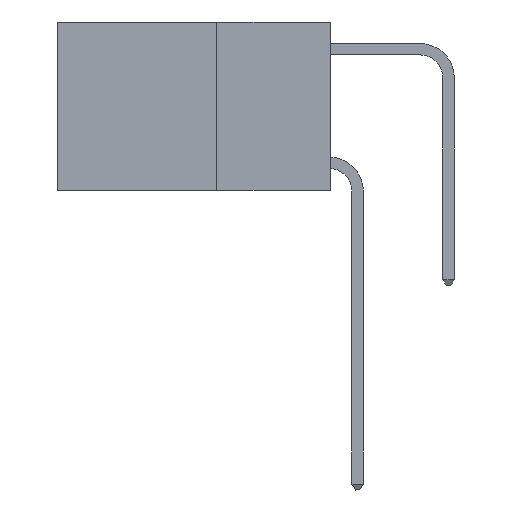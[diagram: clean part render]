
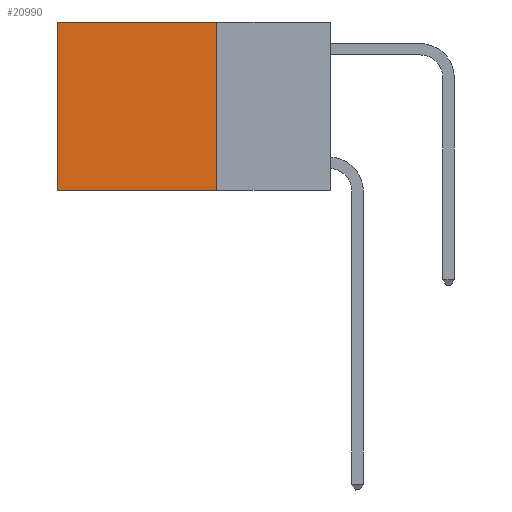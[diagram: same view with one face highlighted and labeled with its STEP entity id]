
A CAD part, left-side view. The second image highlights one B-rep face of the part: STEP entity #20990.
In plain terms, the highlighted planar face has unit normal (-1, 0, 0).
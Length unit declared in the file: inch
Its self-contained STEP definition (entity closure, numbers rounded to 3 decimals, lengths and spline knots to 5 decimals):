
#820 = CARTESIAN_POINT ( 'NONE',  ( 0.2625, 0.25, 0. ) ) ;
#863 = VECTOR ( 'NONE', #4095, 39.37008 ) ;
#1555 = PLANE ( 'NONE',  #19577 ) ;
#2429 = LINE ( 'NONE', #5740, #863 ) ;
#3528 = CARTESIAN_POINT ( 'NONE',  ( 0.2625, 0.6, 0. ) ) ;
#4095 = DIRECTION ( 'NONE',  ( 0., 0., -1. ) ) ;
#4632 = CARTESIAN_POINT ( 'NONE',  ( 0.2625, 0.25, 0. ) ) ;
#4804 = DIRECTION ( 'NONE',  ( 1., 0., 0. ) ) ;
#4837 = VERTEX_POINT ( 'NONE', #3528 ) ;
#5740 = CARTESIAN_POINT ( 'NONE',  ( 0.2625, 0.25, 0. ) ) ;
#6260 = ORIENTED_EDGE ( 'NONE', *, *, #18412, .F. ) ;
#6967 = VERTEX_POINT ( 'NONE', #15767 ) ;
#7458 = EDGE_CURVE ( 'NONE', #9533, #6967, #2429, .T. ) ;
#8333 = CARTESIAN_POINT ( 'NONE',  ( 0.2625, 0.6, -0.37 ) ) ;
#8626 = CARTESIAN_POINT ( 'NONE',  ( 0.2625, 0.25, -0.37 ) ) ;
#9272 = LINE ( 'NONE', #4632, #14155 ) ;
#9335 = ORIENTED_EDGE ( 'NONE', *, *, #7458, .F. ) ;
#9533 = VERTEX_POINT ( 'NONE', #19269 ) ;
#10893 = ORIENTED_EDGE ( 'NONE', *, *, #13325, .T. ) ;
#11121 = LINE ( 'NONE', #12472, #19354 ) ;
#11398 = DIRECTION ( 'NONE',  ( 0., 0., -1. ) ) ;
#11458 = VERTEX_POINT ( 'NONE', #8333 ) ;
#12472 = CARTESIAN_POINT ( 'NONE',  ( 0.2625, 0.6, 0. ) ) ;
#13078 = FACE_OUTER_BOUND ( 'NONE', #17540, .T. ) ;
#13325 = EDGE_CURVE ( 'NONE', #9533, #4837, #9272, .T. ) ;
#13994 = DIRECTION ( 'NONE',  ( 0., 1., 0. ) ) ;
#14007 = VECTOR ( 'NONE', #13994, 39.37008 ) ;
#14155 = VECTOR ( 'NONE', #21208, 39.37008 ) ;
#15283 = ORIENTED_EDGE ( 'NONE', *, *, #18095, .T. ) ;
#15767 = CARTESIAN_POINT ( 'NONE',  ( 0.2625, 0.25, -0.37 ) ) ;
#17540 = EDGE_LOOP ( 'NONE', ( #15283, #6260, #9335, #10893 ) ) ;
#18095 = EDGE_CURVE ( 'NONE', #4837, #11458, #11121, .T. ) ;
#18412 = EDGE_CURVE ( 'NONE', #6967, #11458, #20543, .T. ) ;
#19269 = CARTESIAN_POINT ( 'NONE',  ( 0.2625, 0.25, 0. ) ) ;
#19354 = VECTOR ( 'NONE', #20781, 39.37008 ) ;
#19577 = AXIS2_PLACEMENT_3D ( 'NONE', #820, #4804, #11398 ) ;
#20543 = LINE ( 'NONE', #8626, #14007 ) ;
#20781 = DIRECTION ( 'NONE',  ( 0., 0., -1. ) ) ;
#20990 = ADVANCED_FACE ( 'NONE', ( #13078 ), #1555, .F. ) ;
#21208 = DIRECTION ( 'NONE',  ( 0., 1., 0. ) ) ;
